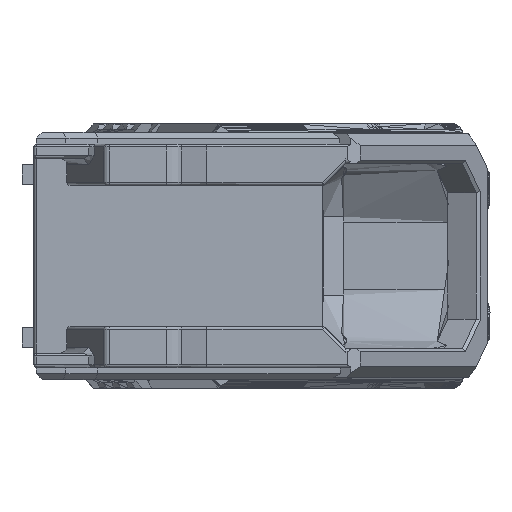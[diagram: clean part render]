
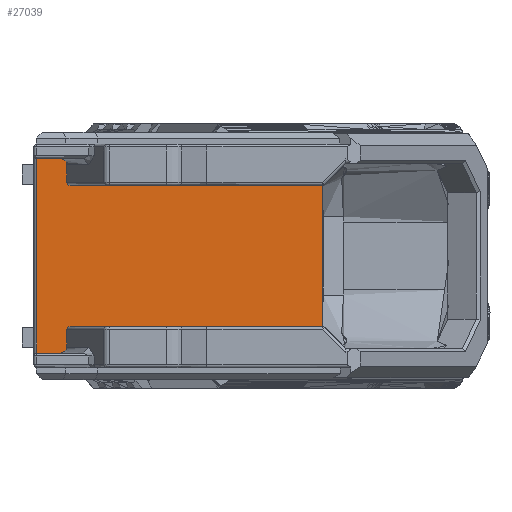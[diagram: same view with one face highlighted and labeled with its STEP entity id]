
A CAD part, left-side view. The second image highlights one B-rep face of the part: STEP entity #27039.
In plain terms, the highlighted planar face has unit normal (-1, 0, 0).
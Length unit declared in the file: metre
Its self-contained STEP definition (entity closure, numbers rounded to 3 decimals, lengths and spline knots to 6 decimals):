
#143=ELLIPSE('',#28963,0.000577,0.0005);
#144=ELLIPSE('',#28964,0.001155,0.001);
#145=ELLIPSE('',#28965,0.001155,0.001);
#146=ELLIPSE('',#28966,0.000577,0.0005);
#599=CIRCLE('',#28946,0.0005);
#602=CIRCLE('',#28951,0.0005);
#2002=ORIENTED_EDGE('',*,*,#9400,.F.);
#2003=ORIENTED_EDGE('',*,*,#9402,.F.);
#2004=ORIENTED_EDGE('',*,*,#9403,.T.);
#2005=ORIENTED_EDGE('',*,*,#9404,.T.);
#2006=ORIENTED_EDGE('',*,*,#9405,.F.);
#2007=ORIENTED_EDGE('',*,*,#9406,.F.);
#2008=ORIENTED_EDGE('',*,*,#9407,.F.);
#2009=ORIENTED_EDGE('',*,*,#9408,.T.);
#2010=ORIENTED_EDGE('',*,*,#9409,.T.);
#2011=ORIENTED_EDGE('',*,*,#9410,.F.);
#2012=ORIENTED_EDGE('',*,*,#9411,.F.);
#2013=ORIENTED_EDGE('',*,*,#9385,.F.);
#2014=ORIENTED_EDGE('',*,*,#9102,.F.);
#2015=ORIENTED_EDGE('',*,*,#9412,.T.);
#2016=ORIENTED_EDGE('',*,*,#9381,.F.);
#2017=ORIENTED_EDGE('',*,*,#9390,.F.);
#9102=EDGE_CURVE('',#12942,#12943,#15116,.T.);
#9381=EDGE_CURVE('',#13126,#13127,#15336,.T.);
#9385=EDGE_CURVE('',#12943,#13130,#599,.T.);
#9390=EDGE_CURVE('',#13132,#13126,#602,.T.);
#9400=EDGE_CURVE('',#13139,#13132,#15345,.T.);
#9402=EDGE_CURVE('',#13140,#13139,#143,.T.);
#9403=EDGE_CURVE('',#13140,#13141,#15346,.T.);
#9404=EDGE_CURVE('',#13141,#13142,#144,.T.);
#9405=EDGE_CURVE('',#13143,#13142,#15347,.T.);
#9406=EDGE_CURVE('',#13144,#13143,#15348,.T.);
#9407=EDGE_CURVE('',#13145,#13144,#15349,.T.);
#9408=EDGE_CURVE('',#13145,#13146,#145,.F.);
#9409=EDGE_CURVE('',#13146,#13147,#15350,.T.);
#9410=EDGE_CURVE('',#13148,#13147,#146,.T.);
#9411=EDGE_CURVE('',#13130,#13148,#15351,.T.);
#9412=EDGE_CURVE('',#12942,#13127,#15352,.T.);
#12942=VERTEX_POINT('',#39412);
#12943=VERTEX_POINT('',#39414);
#13126=VERTEX_POINT('',#40077);
#13127=VERTEX_POINT('',#40079);
#13130=VERTEX_POINT('',#40087);
#13132=VERTEX_POINT('',#40095);
#13139=VERTEX_POINT('',#40115);
#13140=VERTEX_POINT('',#40121);
#13141=VERTEX_POINT('',#40123);
#13142=VERTEX_POINT('',#40125);
#13143=VERTEX_POINT('',#40127);
#13144=VERTEX_POINT('',#40129);
#13145=VERTEX_POINT('',#40131);
#13146=VERTEX_POINT('',#40133);
#13147=VERTEX_POINT('',#40135);
#13148=VERTEX_POINT('',#40137);
#15116=LINE('',#39413,#18512);
#15336=LINE('',#40078,#18732);
#15345=LINE('',#40116,#18741);
#15346=LINE('',#40122,#18742);
#15347=LINE('',#40126,#18743);
#15348=LINE('',#40128,#18744);
#15349=LINE('',#40130,#18745);
#15350=LINE('',#40134,#18746);
#15351=LINE('',#40138,#18747);
#15352=LINE('',#40139,#18748);
#18512=VECTOR('',#31490,1.);
#18732=VECTOR('',#31978,1.);
#18741=VECTOR('',#32019,1.);
#18742=VECTOR('',#32028,1.);
#18743=VECTOR('',#32031,1.);
#18744=VECTOR('',#32032,1.);
#18745=VECTOR('',#32033,1.);
#18746=VECTOR('',#32036,1.);
#18747=VECTOR('',#32039,1.);
#18748=VECTOR('',#32040,1.);
#21647=EDGE_LOOP('',(#2002,#2003,#2004,#2005,#2006,#2007,#2008,#2009,#2010,
#2011,#2012,#2013,#2014,#2015,#2016,#2017));
#23511=FACE_BOUND('',#21647,.T.);
#25348=PLANE('',#28962);
#27039=ADVANCED_FACE('',(#23511),#25348,.F.);
#28946=AXIS2_PLACEMENT_3D('',#40086,#31985,#31986);
#28951=AXIS2_PLACEMENT_3D('',#40096,#31997,#31998);
#28962=AXIS2_PLACEMENT_3D('',#40119,#32024,#32025);
#28963=AXIS2_PLACEMENT_3D('',#40120,#32026,#32027);
#28964=AXIS2_PLACEMENT_3D('',#40124,#32029,#32030);
#28965=AXIS2_PLACEMENT_3D('',#40132,#32034,#32035);
#28966=AXIS2_PLACEMENT_3D('',#40136,#32037,#32038);
#31490=DIRECTION('',(0.,-0.707,-0.707));
#31978=DIRECTION('',(0.,0.707,-0.707));
#31985=DIRECTION('',(-1.,0.,0.));
#31986=DIRECTION('',(0.,-0.383,0.924));
#31997=DIRECTION('',(-1.,0.,0.));
#31998=DIRECTION('',(0.,-0.383,-0.924));
#32019=DIRECTION('',(0.,-1.,0.));
#32024=DIRECTION('',(1.,0.,0.));
#32025=DIRECTION('',(0.,0.,-1.));
#32026=DIRECTION('',(-1.,0.,0.));
#32027=DIRECTION('',(0.,1.,0.));
#32028=DIRECTION('',(0.,0.,1.));
#32029=DIRECTION('',(-1.,0.,0.));
#32030=DIRECTION('',(0.,1.,0.));
#32031=DIRECTION('',(0.,-1.,0.));
#32032=DIRECTION('',(0.,0.,1.));
#32033=DIRECTION('',(0.,1.,0.));
#32034=DIRECTION('',(1.,0.,0.));
#32035=DIRECTION('',(0.,1.,0.));
#32036=DIRECTION('',(0.,0.,1.));
#32037=DIRECTION('',(-1.,0.,0.));
#32038=DIRECTION('',(0.,1.,0.));
#32039=DIRECTION('',(0.,1.,0.));
#32040=DIRECTION('',(0.,0.,1.));
#39412=CARTESIAN_POINT('',(-0.0824,-0.05729,-0.01075));
#39413=CARTESIAN_POINT('',(-0.0824,-0.048815,-0.002275));
#39414=CARTESIAN_POINT('',(-0.0824,-0.057686,-0.011146));
#40077=CARTESIAN_POINT('',(-0.0824,-0.057686,0.013146));
#40078=CARTESIAN_POINT('',(-0.0824,-0.048815,0.004275));
#40079=CARTESIAN_POINT('',(-0.0824,-0.05729,0.01275));
#40086=CARTESIAN_POINT('',(-0.0824,-0.057332,-0.0115));
#40087=CARTESIAN_POINT('',(-0.0824,-0.057332,-0.011));
#40095=CARTESIAN_POINT('',(-0.0824,-0.057333,0.013));
#40096=CARTESIAN_POINT('',(-0.0824,-0.057333,0.0135));
#40115=CARTESIAN_POINT('',(-0.0824,-0.014485,0.013));
#40116=CARTESIAN_POINT('',(-0.0824,-0.03284,0.013));
#40119=CARTESIAN_POINT('',(-0.0824,-0.031141,0.001));
#40120=CARTESIAN_POINT('',(-0.0824,-0.014485,0.0135));
#40121=CARTESIAN_POINT('',(-0.0824,-0.013907,0.0135));
#40122=CARTESIAN_POINT('',(-0.0824,-0.013907,-0.0091));
#40123=CARTESIAN_POINT('',(-0.0824,-0.013907,0.0165));
#40124=CARTESIAN_POINT('',(-0.0824,-0.012753,0.0165));
#40125=CARTESIAN_POINT('',(-0.0824,-0.012753,0.0175));
#40126=CARTESIAN_POINT('',(-0.0824,-0.03284,0.0175));
#40127=CARTESIAN_POINT('',(-0.0824,-0.00879,0.0175));
#40128=CARTESIAN_POINT('',(-0.0824,-0.00879,0.001));
#40129=CARTESIAN_POINT('',(-0.0824,-0.00879,-0.0155));
#40130=CARTESIAN_POINT('',(-0.0824,-0.031953,-0.0155));
#40131=CARTESIAN_POINT('',(-0.0824,-0.012753,-0.0155));
#40132=CARTESIAN_POINT('',(-0.0824,-0.012753,-0.0145));
#40133=CARTESIAN_POINT('',(-0.0824,-0.013907,-0.0145));
#40134=CARTESIAN_POINT('',(-0.0824,-0.013907,-0.0091));
#40135=CARTESIAN_POINT('',(-0.0824,-0.013907,-0.0115));
#40136=CARTESIAN_POINT('',(-0.0824,-0.014485,-0.0115));
#40137=CARTESIAN_POINT('',(-0.0824,-0.014485,-0.011));
#40138=CARTESIAN_POINT('',(-0.0824,-0.031547,-0.011));
#40139=CARTESIAN_POINT('',(-0.0824,-0.05729,0.00917));
